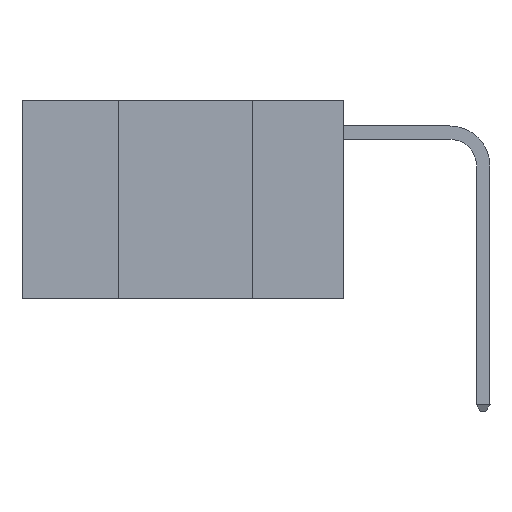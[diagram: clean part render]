
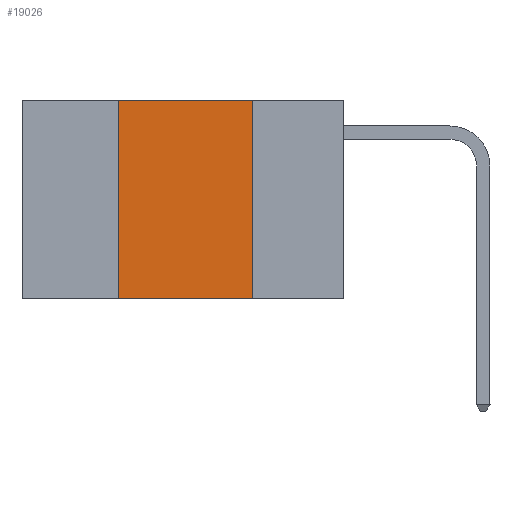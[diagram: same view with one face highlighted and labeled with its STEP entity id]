
A CAD part, left-side view. The second image highlights one B-rep face of the part: STEP entity #19026.
In plain terms, the highlighted planar face has unit normal (-1, 0, 0).
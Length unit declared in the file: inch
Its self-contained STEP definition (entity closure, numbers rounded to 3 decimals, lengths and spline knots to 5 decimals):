
#68 = DIRECTION ( 'NONE',  ( 1., 0., 0. ) ) ;
#3361 = CARTESIAN_POINT ( 'NONE',  ( 0., 0.17, 0. ) ) ;
#3723 = LINE ( 'NONE', #28072, #20389 ) ;
#3799 = DIRECTION ( 'NONE',  ( 0., -1., 0. ) ) ;
#3984 = CARTESIAN_POINT ( 'NONE',  ( 0., 0.17, 0. ) ) ;
#5029 = AXIS2_PLACEMENT_3D ( 'NONE', #23970, #68, #15423 ) ;
#5036 = EDGE_CURVE ( 'NONE', #19517, #10009, #5119, .T. ) ;
#5119 = LINE ( 'NONE', #3361, #18795 ) ;
#6322 = CARTESIAN_POINT ( 'NONE',  ( 0., 0.42, -0.37 ) ) ;
#6808 = DIRECTION ( 'NONE',  ( 0., 0., 1. ) ) ;
#7668 = EDGE_CURVE ( 'NONE', #16264, #19517, #27550, .T. ) ;
#8179 = VECTOR ( 'NONE', #19217, 39.37008 ) ;
#8185 = EDGE_CURVE ( 'NONE', #20185, #10009, #14645, .T. ) ;
#8334 = ORIENTED_EDGE ( 'NONE', *, *, #5036, .F. ) ;
#10009 = VERTEX_POINT ( 'NONE', #16876 ) ;
#10277 = EDGE_LOOP ( 'NONE', ( #8334, #19856, #15500, #26993 ) ) ;
#14645 = LINE ( 'NONE', #14868, #8179 ) ;
#14706 = CARTESIAN_POINT ( 'NONE',  ( 0., 0.6, 0. ) ) ;
#14868 = CARTESIAN_POINT ( 'NONE',  ( 0., 0.6, -0.37 ) ) ;
#15423 = DIRECTION ( 'NONE',  ( 0., 0., -1. ) ) ;
#15500 = ORIENTED_EDGE ( 'NONE', *, *, #25617, .F. ) ;
#16054 = VECTOR ( 'NONE', #3799, 39.37008 ) ;
#16264 = VERTEX_POINT ( 'NONE', #25791 ) ;
#16876 = CARTESIAN_POINT ( 'NONE',  ( 0., 0.17, -0.37 ) ) ;
#17505 = PLANE ( 'NONE',  #5029 ) ;
#18795 = VECTOR ( 'NONE', #25128, 39.37008 ) ;
#19026 = ADVANCED_FACE ( 'NONE', ( #25465 ), #17505, .F. ) ;
#19217 = DIRECTION ( 'NONE',  ( 0., -1., 0. ) ) ;
#19517 = VERTEX_POINT ( 'NONE', #3984 ) ;
#19856 = ORIENTED_EDGE ( 'NONE', *, *, #7668, .F. ) ;
#20185 = VERTEX_POINT ( 'NONE', #6322 ) ;
#20389 = VECTOR ( 'NONE', #6808, 39.37008 ) ;
#23970 = CARTESIAN_POINT ( 'NONE',  ( 0., 0.6, 0. ) ) ;
#25128 = DIRECTION ( 'NONE',  ( 0., 0., -1. ) ) ;
#25465 = FACE_OUTER_BOUND ( 'NONE', #10277, .T. ) ;
#25617 = EDGE_CURVE ( 'NONE', #20185, #16264, #3723, .T. ) ;
#25791 = CARTESIAN_POINT ( 'NONE',  ( 0., 0.42, 0. ) ) ;
#26993 = ORIENTED_EDGE ( 'NONE', *, *, #8185, .T. ) ;
#27550 = LINE ( 'NONE', #14706, #16054 ) ;
#28072 = CARTESIAN_POINT ( 'NONE',  ( 0., 0.42, 0. ) ) ;
